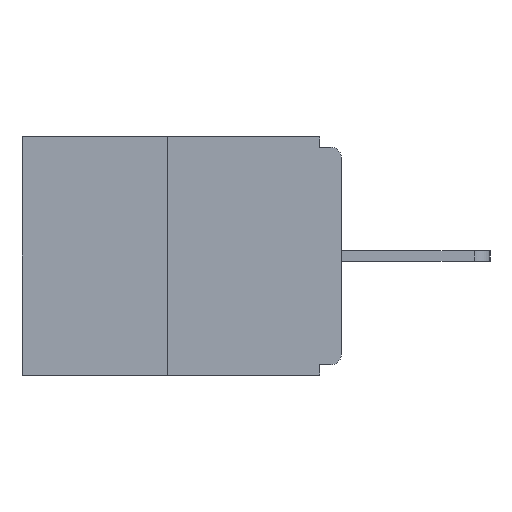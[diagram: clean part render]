
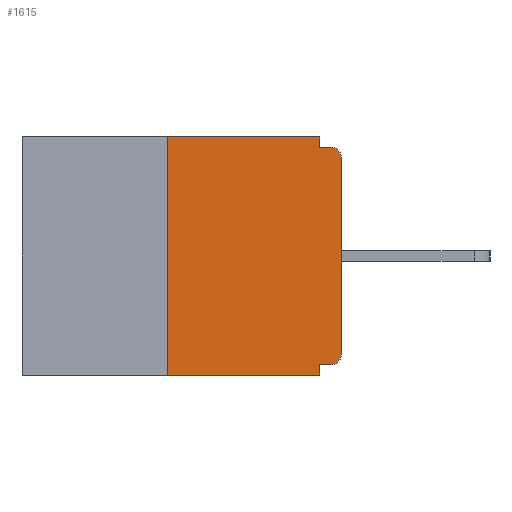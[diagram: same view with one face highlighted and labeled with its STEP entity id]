
A CAD part, left-side view. The second image highlights one B-rep face of the part: STEP entity #1615.
In plain terms, the highlighted planar face has unit normal (-1, 0, 0).
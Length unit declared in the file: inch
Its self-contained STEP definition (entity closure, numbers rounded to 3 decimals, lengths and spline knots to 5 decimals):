
#51 = VERTEX_POINT ( 'NONE', #2752 ) ;
#270 = VERTEX_POINT ( 'NONE', #2098 ) ;
#372 = CARTESIAN_POINT ( 'NONE',  ( 0., 0.015, -0.03 ) ) ;
#441 = VECTOR ( 'NONE', #7066, 39.37008 ) ;
#608 = ORIENTED_EDGE ( 'NONE', *, *, #3807, .F. ) ;
#710 = EDGE_CURVE ( 'NONE', #9101, #51, #1255, .T. ) ;
#730 = ORIENTED_EDGE ( 'NONE', *, *, #8991, .F. ) ;
#1132 = CARTESIAN_POINT ( 'NONE',  ( 0., 0., -0.313 ) ) ;
#1150 = PLANE ( 'NONE',  #13158 ) ;
#1255 = LINE ( 'NONE', #13403, #10692 ) ;
#1339 = DIRECTION ( 'NONE',  ( 0., -1., 0. ) ) ;
#1546 = EDGE_CURVE ( 'NONE', #5743, #10034, #11466, .T. ) ;
#1615 = ADVANCED_FACE ( 'NONE', ( #3503 ), #1150, .F. ) ;
#1718 = CARTESIAN_POINT ( 'NONE',  ( 0., 0., -0.328 ) ) ;
#2098 = CARTESIAN_POINT ( 'NONE',  ( 0., 0.25, -0.343 ) ) ;
#2140 = EDGE_CURVE ( 'NONE', #11674, #6592, #11959, .T. ) ;
#2249 = DIRECTION ( 'NONE',  ( 0., 0., -1. ) ) ;
#2485 = AXIS2_PLACEMENT_3D ( 'NONE', #372, #8680, #5546 ) ;
#2579 = AXIS2_PLACEMENT_3D ( 'NONE', #6024, #10161, #12215 ) ;
#2752 = CARTESIAN_POINT ( 'NONE',  ( 0., 0.031, -0.343 ) ) ;
#2986 = VECTOR ( 'NONE', #8639, 39.37008 ) ;
#3117 = LINE ( 'NONE', #1718, #441 ) ;
#3251 = CARTESIAN_POINT ( 'NONE',  ( 0., 0.25, 0. ) ) ;
#3503 = FACE_OUTER_BOUND ( 'NONE', #11146, .T. ) ;
#3545 = EDGE_CURVE ( 'NONE', #270, #51, #11394, .T. ) ;
#3601 = DIRECTION ( 'NONE',  ( 0., -1., 0. ) ) ;
#3807 = EDGE_CURVE ( 'NONE', #10034, #12336, #10244, .T. ) ;
#3858 = VERTEX_POINT ( 'NONE', #10045 ) ;
#3944 = ORIENTED_EDGE ( 'NONE', *, *, #12548, .T. ) ;
#4106 = CARTESIAN_POINT ( 'NONE',  ( 0., 0.015, -0.328 ) ) ;
#4354 = ORIENTED_EDGE ( 'NONE', *, *, #710, .F. ) ;
#4436 = ORIENTED_EDGE ( 'NONE', *, *, #13023, .F. ) ;
#4634 = CARTESIAN_POINT ( 'NONE',  ( 0., 0., -0.015 ) ) ;
#4767 = VECTOR ( 'NONE', #12434, 39.37008 ) ;
#5017 = CARTESIAN_POINT ( 'NONE',  ( 0., 0.46, -0.343 ) ) ;
#5042 = ORIENTED_EDGE ( 'NONE', *, *, #1546, .F. ) ;
#5195 = VERTEX_POINT ( 'NONE', #4106 ) ;
#5546 = DIRECTION ( 'NONE',  ( 0., 0., -1. ) ) ;
#5547 = CARTESIAN_POINT ( 'NONE',  ( 0., 0.46, 0. ) ) ;
#5727 = CARTESIAN_POINT ( 'NONE',  ( 0., 0.031, -0.015 ) ) ;
#5743 = VERTEX_POINT ( 'NONE', #7062 ) ;
#6024 = CARTESIAN_POINT ( 'NONE',  ( 0., 0.015, -0.313 ) ) ;
#6453 = CIRCLE ( 'NONE', #2485, 0.015 ) ;
#6528 = CARTESIAN_POINT ( 'NONE',  ( 0., 0.031, -0.328 ) ) ;
#6578 = CARTESIAN_POINT ( 'NONE',  ( 0., 0.46, 0. ) ) ;
#6592 = VERTEX_POINT ( 'NONE', #11923 ) ;
#6764 = LINE ( 'NONE', #5547, #11550 ) ;
#7062 = CARTESIAN_POINT ( 'NONE',  ( 0., 0.031, 0. ) ) ;
#7066 = DIRECTION ( 'NONE',  ( 0., 1., 0. ) ) ;
#7496 = VECTOR ( 'NONE', #11524, 39.37008 ) ;
#8002 = ORIENTED_EDGE ( 'NONE', *, *, #10840, .T. ) ;
#8154 = DIRECTION ( 'NONE',  ( 0., 0., -1. ) ) ;
#8223 = ORIENTED_EDGE ( 'NONE', *, *, #12533, .F. ) ;
#8384 = DIRECTION ( 'NONE',  ( 0., 0., 1. ) ) ;
#8536 = DIRECTION ( 'NONE',  ( 1., 0., 0. ) ) ;
#8639 = DIRECTION ( 'NONE',  ( 0., 0., 1. ) ) ;
#8680 = DIRECTION ( 'NONE',  ( -1., 0., 0. ) ) ;
#8991 = EDGE_CURVE ( 'NONE', #270, #3858, #11781, .T. ) ;
#9101 = VERTEX_POINT ( 'NONE', #6528 ) ;
#9391 = CARTESIAN_POINT ( 'NONE',  ( 0., 0.031, 0. ) ) ;
#9595 = CARTESIAN_POINT ( 'NONE',  ( 0., 0., 0. ) ) ;
#10034 = VERTEX_POINT ( 'NONE', #5727 ) ;
#10045 = CARTESIAN_POINT ( 'NONE',  ( 0., 0.25, 0. ) ) ;
#10161 = DIRECTION ( 'NONE',  ( -1., 0., 0. ) ) ;
#10244 = LINE ( 'NONE', #4634, #10395 ) ;
#10395 = VECTOR ( 'NONE', #3601, 39.37008 ) ;
#10564 = CIRCLE ( 'NONE', #2579, 0.015 ) ;
#10692 = VECTOR ( 'NONE', #8154, 39.37008 ) ;
#10840 = EDGE_CURVE ( 'NONE', #6592, #12336, #6453, .T. ) ;
#11146 = EDGE_LOOP ( 'NONE', ( #4436, #730, #12869, #4354, #8223, #3944, #12059, #8002, #608, #5042 ) ) ;
#11394 = LINE ( 'NONE', #5017, #4767 ) ;
#11466 = LINE ( 'NONE', #9391, #7496 ) ;
#11524 = DIRECTION ( 'NONE',  ( 0., 0., -1. ) ) ;
#11550 = VECTOR ( 'NONE', #1339, 39.37008 ) ;
#11674 = VERTEX_POINT ( 'NONE', #1132 ) ;
#11781 = LINE ( 'NONE', #3251, #13148 ) ;
#11923 = CARTESIAN_POINT ( 'NONE',  ( 0., 0., -0.03 ) ) ;
#11959 = LINE ( 'NONE', #9595, #2986 ) ;
#12059 = ORIENTED_EDGE ( 'NONE', *, *, #2140, .T. ) ;
#12215 = DIRECTION ( 'NONE',  ( 0., 0., -1. ) ) ;
#12336 = VERTEX_POINT ( 'NONE', #12977 ) ;
#12434 = DIRECTION ( 'NONE',  ( 0., -1., 0. ) ) ;
#12533 = EDGE_CURVE ( 'NONE', #5195, #9101, #3117, .T. ) ;
#12548 = EDGE_CURVE ( 'NONE', #5195, #11674, #10564, .T. ) ;
#12869 = ORIENTED_EDGE ( 'NONE', *, *, #3545, .T. ) ;
#12977 = CARTESIAN_POINT ( 'NONE',  ( 0., 0.015, -0.015 ) ) ;
#13023 = EDGE_CURVE ( 'NONE', #3858, #5743, #6764, .T. ) ;
#13148 = VECTOR ( 'NONE', #8384, 39.37008 ) ;
#13158 = AXIS2_PLACEMENT_3D ( 'NONE', #6578, #8536, #2249 ) ;
#13403 = CARTESIAN_POINT ( 'NONE',  ( 0., 0.031, -0.343 ) ) ;
